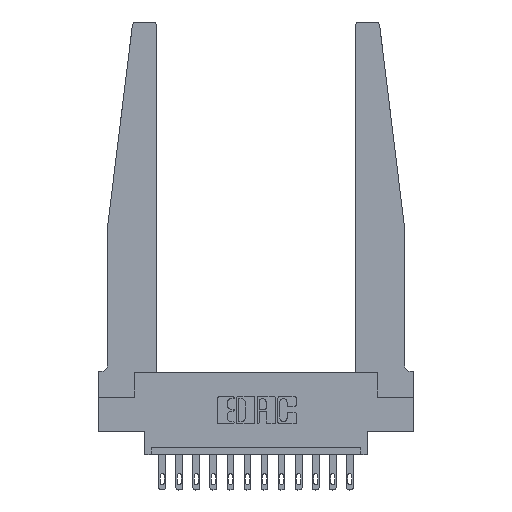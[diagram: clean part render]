
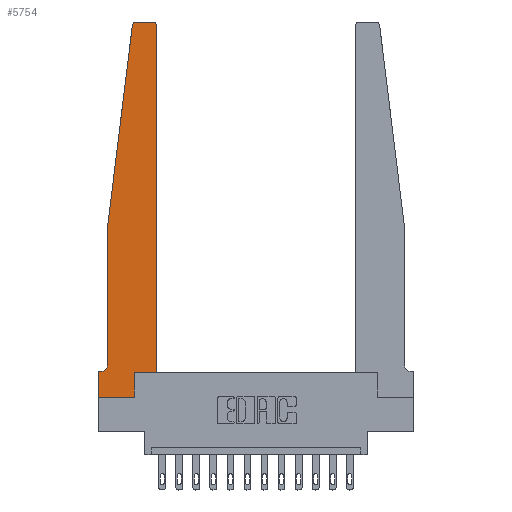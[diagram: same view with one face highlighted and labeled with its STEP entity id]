
A CAD part, top view. The second image highlights one B-rep face of the part: STEP entity #5754.
In plain terms, the highlighted planar face has unit normal (0, 0, 1).
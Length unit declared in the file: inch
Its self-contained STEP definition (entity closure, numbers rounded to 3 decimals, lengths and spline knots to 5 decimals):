
#90 = CARTESIAN_POINT ( 'NONE',  ( 0.065, 1.25, 0.37 ) ) ;
#94 = CIRCLE ( 'NONE', #11272, 0.03 ) ;
#749 = DIRECTION ( 'NONE',  ( 1., 0., 0. ) ) ;
#851 = CARTESIAN_POINT ( 'NONE',  ( 0.2605, 0., 0.37 ) ) ;
#909 = CARTESIAN_POINT ( 'NONE',  ( 0.065, 1.25, 0.37 ) ) ;
#1129 = CARTESIAN_POINT ( 'NONE',  ( 0.065, 1.25, 0.37 ) ) ;
#1235 = CIRCLE ( 'NONE', #2579, 0.03 ) ;
#1312 = EDGE_CURVE ( 'NONE', #14408, #12777, #94, .T. ) ;
#1327 = CARTESIAN_POINT ( 'NONE',  ( 0.2605, 0.18, 0.37 ) ) ;
#1611 = VECTOR ( 'NONE', #3600, 39.37008 ) ;
#1904 = DIRECTION ( 'NONE',  ( 0., 0., 1. ) ) ;
#1912 = LINE ( 'NONE', #5974, #14729 ) ;
#2200 = EDGE_CURVE ( 'NONE', #12777, #15618, #14661, .T. ) ;
#2428 = VERTEX_POINT ( 'NONE', #851 ) ;
#2579 = AXIS2_PLACEMENT_3D ( 'NONE', #11104, #1904, #16053 ) ;
#2725 = VECTOR ( 'NONE', #9804, 39.37008 ) ;
#2766 = CARTESIAN_POINT ( 'NONE',  ( 0.2605, 0.18, 0.37 ) ) ;
#2783 = EDGE_CURVE ( 'NONE', #15608, #14408, #6475, .T. ) ;
#2957 = VERTEX_POINT ( 'NONE', #15873 ) ;
#3044 = ORIENTED_EDGE ( 'NONE', *, *, #11380, .T. ) ;
#3090 = ORIENTED_EDGE ( 'NONE', *, *, #2200, .T. ) ;
#3349 = CARTESIAN_POINT ( 'NONE',  ( 0.015, 0.1875, 0.37 ) ) ;
#3600 = DIRECTION ( 'NONE',  ( -1., 0., 0. ) ) ;
#3742 = CARTESIAN_POINT ( 'NONE',  ( 0.395, 2.75, 0.37 ) ) ;
#3940 = CARTESIAN_POINT ( 'NONE',  ( 0.25, 2.75, 0.37 ) ) ;
#4618 = CARTESIAN_POINT ( 'NONE',  ( 0.425, 0.18, 0.37 ) ) ;
#4677 = CARTESIAN_POINT ( 'NONE',  ( 0.425, 0.18, 0.37 ) ) ;
#4794 = CARTESIAN_POINT ( 'NONE',  ( 0.27653, 2.75, 0.37 ) ) ;
#5140 = CARTESIAN_POINT ( 'NONE',  ( 0., 0., 0.37 ) ) ;
#5383 = VERTEX_POINT ( 'NONE', #5140 ) ;
#5710 = AXIS2_PLACEMENT_3D ( 'NONE', #12390, #13697, #749 ) ;
#5754 = ADVANCED_FACE ( 'NONE', ( #5899 ), #9819, .T. ) ;
#5877 = ORIENTED_EDGE ( 'NONE', *, *, #6675, .T. ) ;
#5899 = FACE_OUTER_BOUND ( 'NONE', #9140, .T. ) ;
#5974 = CARTESIAN_POINT ( 'NONE',  ( 0.065, 0.1875, 0.37 ) ) ;
#6084 = CARTESIAN_POINT ( 'NONE',  ( 0., 0., 0.37 ) ) ;
#6173 = CARTESIAN_POINT ( 'NONE',  ( 0.27653, 2.72, 0.37 ) ) ;
#6475 = LINE ( 'NONE', #3940, #1611 ) ;
#6485 = ORIENTED_EDGE ( 'NONE', *, *, #11066, .T. ) ;
#6499 = EDGE_CURVE ( 'NONE', #12692, #5383, #13721, .T. ) ;
#6506 = ORIENTED_EDGE ( 'NONE', *, *, #8246, .T. ) ;
#6675 = EDGE_CURVE ( 'NONE', #12819, #12979, #11144, .T. ) ;
#6766 = DIRECTION ( 'NONE',  ( -0.122, -0.992, 0. ) ) ;
#6821 = VECTOR ( 'NONE', #15819, 39.37008 ) ;
#6907 = CARTESIAN_POINT ( 'NONE',  ( 0.065, 0.2375, 0.37 ) ) ;
#7037 = AXIS2_PLACEMENT_3D ( 'NONE', #10606, #15478, #10427 ) ;
#7526 = CARTESIAN_POINT ( 'NONE',  ( 0., 0., 0.37 ) ) ;
#7604 = LINE ( 'NONE', #7526, #16049 ) ;
#8246 = EDGE_CURVE ( 'NONE', #15618, #12819, #10069, .T. ) ;
#8581 = ORIENTED_EDGE ( 'NONE', *, *, #2783, .T. ) ;
#8976 = DIRECTION ( 'NONE',  ( 1., 0., 0. ) ) ;
#9133 = ORIENTED_EDGE ( 'NONE', *, *, #6499, .T. ) ;
#9140 = EDGE_LOOP ( 'NONE', ( #8581, #15298, #3090, #6506, #5877, #11753, #9133, #3044, #12547, #11418, #6485, #13791 ) ) ;
#9305 = CARTESIAN_POINT ( 'NONE',  ( 0.24675, 2.72367, 0.37 ) ) ;
#9324 = CARTESIAN_POINT ( 'NONE',  ( 0.425, 0.18, 0.37 ) ) ;
#9582 = EDGE_CURVE ( 'NONE', #12606, #10444, #9723, .T. ) ;
#9723 = LINE ( 'NONE', #4618, #2725 ) ;
#9804 = DIRECTION ( 'NONE',  ( 1., 0., 0. ) ) ;
#9819 = PLANE ( 'NONE',  #5710 ) ;
#10069 = LINE ( 'NONE', #909, #13229 ) ;
#10427 = DIRECTION ( 'NONE',  ( -1., 0., 0. ) ) ;
#10444 = VERTEX_POINT ( 'NONE', #4677 ) ;
#10606 = CARTESIAN_POINT ( 'NONE',  ( 0.015, 0.2375, 0.37 ) ) ;
#11066 = EDGE_CURVE ( 'NONE', #10444, #2957, #13222, .T. ) ;
#11104 = CARTESIAN_POINT ( 'NONE',  ( 0.395, 2.72, 0.37 ) ) ;
#11144 = CIRCLE ( 'NONE', #7037, 0.05 ) ;
#11217 = DIRECTION ( 'NONE',  ( 0., -1., 0. ) ) ;
#11272 = AXIS2_PLACEMENT_3D ( 'NONE', #6173, #11391, #8976 ) ;
#11376 = DIRECTION ( 'NONE',  ( 1., 0., 0. ) ) ;
#11380 = EDGE_CURVE ( 'NONE', #5383, #2428, #7604, .T. ) ;
#11391 = DIRECTION ( 'NONE',  ( 0., 0., 1. ) ) ;
#11418 = ORIENTED_EDGE ( 'NONE', *, *, #9582, .T. ) ;
#11712 = DIRECTION ( 'NONE',  ( 0., 1., 0. ) ) ;
#11753 = ORIENTED_EDGE ( 'NONE', *, *, #12926, .T. ) ;
#11830 = VECTOR ( 'NONE', #11712, 39.37008 ) ;
#12390 = CARTESIAN_POINT ( 'NONE',  ( 0., 0.1875, 0.37 ) ) ;
#12547 = ORIENTED_EDGE ( 'NONE', *, *, #14726, .T. ) ;
#12606 = VERTEX_POINT ( 'NONE', #1327 ) ;
#12692 = VERTEX_POINT ( 'NONE', #16561 ) ;
#12777 = VERTEX_POINT ( 'NONE', #9305 ) ;
#12819 = VERTEX_POINT ( 'NONE', #6907 ) ;
#12926 = EDGE_CURVE ( 'NONE', #12979, #12692, #1912, .T. ) ;
#12979 = VERTEX_POINT ( 'NONE', #3349 ) ;
#13222 = LINE ( 'NONE', #9324, #6821 ) ;
#13229 = VECTOR ( 'NONE', #13864, 39.37008 ) ;
#13456 = VECTOR ( 'NONE', #6766, 39.37008 ) ;
#13689 = DIRECTION ( 'NONE',  ( -1., 0., 0. ) ) ;
#13697 = DIRECTION ( 'NONE',  ( 0., 0., 1. ) ) ;
#13721 = LINE ( 'NONE', #6084, #16256 ) ;
#13791 = ORIENTED_EDGE ( 'NONE', *, *, #16493, .T. ) ;
#13864 = DIRECTION ( 'NONE',  ( 0., -1., 0. ) ) ;
#14377 = LINE ( 'NONE', #2766, #11830 ) ;
#14408 = VERTEX_POINT ( 'NONE', #4794 ) ;
#14661 = LINE ( 'NONE', #90, #13456 ) ;
#14726 = EDGE_CURVE ( 'NONE', #2428, #12606, #14377, .T. ) ;
#14729 = VECTOR ( 'NONE', #13689, 39.37008 ) ;
#15298 = ORIENTED_EDGE ( 'NONE', *, *, #1312, .T. ) ;
#15478 = DIRECTION ( 'NONE',  ( 0., 0., -1. ) ) ;
#15608 = VERTEX_POINT ( 'NONE', #3742 ) ;
#15618 = VERTEX_POINT ( 'NONE', #1129 ) ;
#15819 = DIRECTION ( 'NONE',  ( 0., 1., 0. ) ) ;
#15873 = CARTESIAN_POINT ( 'NONE',  ( 0.425, 2.72, 0.37 ) ) ;
#16049 = VECTOR ( 'NONE', #11376, 39.37008 ) ;
#16053 = DIRECTION ( 'NONE',  ( 1., 0., 0. ) ) ;
#16256 = VECTOR ( 'NONE', #11217, 39.37008 ) ;
#16493 = EDGE_CURVE ( 'NONE', #2957, #15608, #1235, .T. ) ;
#16561 = CARTESIAN_POINT ( 'NONE',  ( 0., 0.1875, 0.37 ) ) ;
